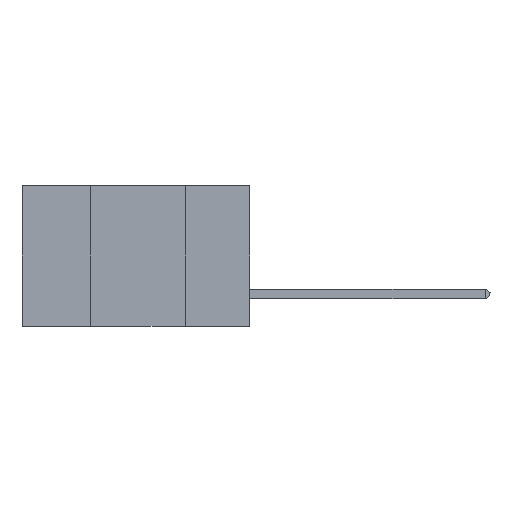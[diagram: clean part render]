
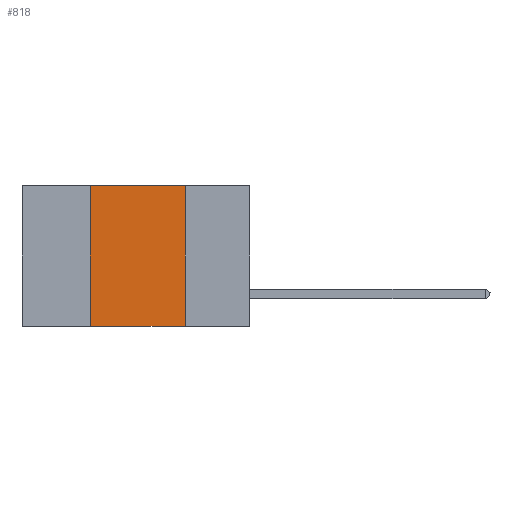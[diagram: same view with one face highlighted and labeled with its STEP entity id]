
A CAD part, left-side view. The second image highlights one B-rep face of the part: STEP entity #818.
In plain terms, the highlighted planar face has unit normal (-1, 0, 0).
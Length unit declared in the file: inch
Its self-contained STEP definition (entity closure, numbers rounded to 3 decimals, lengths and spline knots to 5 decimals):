
#89 = LINE ( 'NONE', #7548, #11928 ) ;
#818 = ADVANCED_FACE ( 'NONE', ( #9153 ), #9735, .F. ) ;
#1879 = CARTESIAN_POINT ( 'NONE',  ( 0., 0.6, -0.37 ) ) ;
#1934 = ORIENTED_EDGE ( 'NONE', *, *, #6042, .F. ) ;
#1943 = LINE ( 'NONE', #10981, #6209 ) ;
#2046 = VERTEX_POINT ( 'NONE', #3646 ) ;
#3168 = DIRECTION ( 'NONE',  ( 0., 0., 1. ) ) ;
#3646 = CARTESIAN_POINT ( 'NONE',  ( 0., 0.17, -0.37 ) ) ;
#5120 = ORIENTED_EDGE ( 'NONE', *, *, #8126, .F. ) ;
#5927 = CARTESIAN_POINT ( 'NONE',  ( 0., 0.42, -0.37 ) ) ;
#6042 = EDGE_CURVE ( 'NONE', #12271, #6181, #1943, .T. ) ;
#6161 = VECTOR ( 'NONE', #9777, 39.37008 ) ;
#6181 = VERTEX_POINT ( 'NONE', #7139 ) ;
#6209 = VECTOR ( 'NONE', #3168, 39.37008 ) ;
#7139 = CARTESIAN_POINT ( 'NONE',  ( 0., 0.42, 0. ) ) ;
#7437 = VERTEX_POINT ( 'NONE', #12161 ) ;
#7495 = LINE ( 'NONE', #1879, #6161 ) ;
#7548 = CARTESIAN_POINT ( 'NONE',  ( 0., 0.17, 0. ) ) ;
#7632 = EDGE_CURVE ( 'NONE', #7437, #2046, #89, .T. ) ;
#8126 = EDGE_CURVE ( 'NONE', #6181, #7437, #11306, .T. ) ;
#8871 = DIRECTION ( 'NONE',  ( 0., 0., -1. ) ) ;
#9153 = FACE_OUTER_BOUND ( 'NONE', #11574, .T. ) ;
#9597 = DIRECTION ( 'NONE',  ( 1., 0., 0. ) ) ;
#9735 = PLANE ( 'NONE',  #11157 ) ;
#9777 = DIRECTION ( 'NONE',  ( 0., -1., 0. ) ) ;
#10681 = CARTESIAN_POINT ( 'NONE',  ( 0., 0.6, 0. ) ) ;
#10974 = ORIENTED_EDGE ( 'NONE', *, *, #11597, .T. ) ;
#10981 = CARTESIAN_POINT ( 'NONE',  ( 0., 0.42, 0. ) ) ;
#11125 = CARTESIAN_POINT ( 'NONE',  ( 0., 0.6, 0. ) ) ;
#11157 = AXIS2_PLACEMENT_3D ( 'NONE', #10681, #9597, #8871 ) ;
#11306 = LINE ( 'NONE', #11125, #11636 ) ;
#11574 = EDGE_LOOP ( 'NONE', ( #12190, #5120, #1934, #10974 ) ) ;
#11597 = EDGE_CURVE ( 'NONE', #12271, #2046, #7495, .T. ) ;
#11636 = VECTOR ( 'NONE', #12090, 39.37008 ) ;
#11928 = VECTOR ( 'NONE', #12401, 39.37008 ) ;
#12090 = DIRECTION ( 'NONE',  ( 0., -1., 0. ) ) ;
#12161 = CARTESIAN_POINT ( 'NONE',  ( 0., 0.17, 0. ) ) ;
#12190 = ORIENTED_EDGE ( 'NONE', *, *, #7632, .F. ) ;
#12271 = VERTEX_POINT ( 'NONE', #5927 ) ;
#12401 = DIRECTION ( 'NONE',  ( 0., 0., -1. ) ) ;
